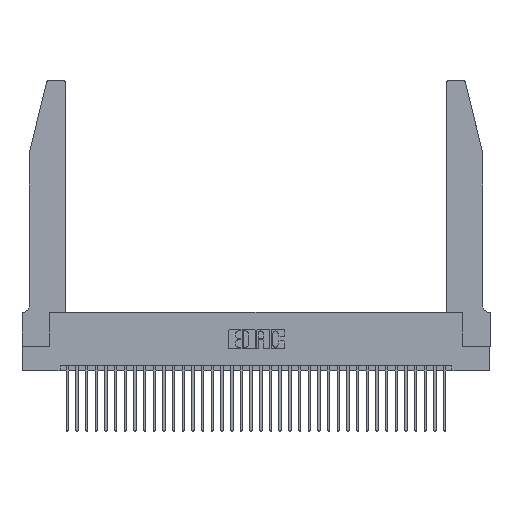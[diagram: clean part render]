
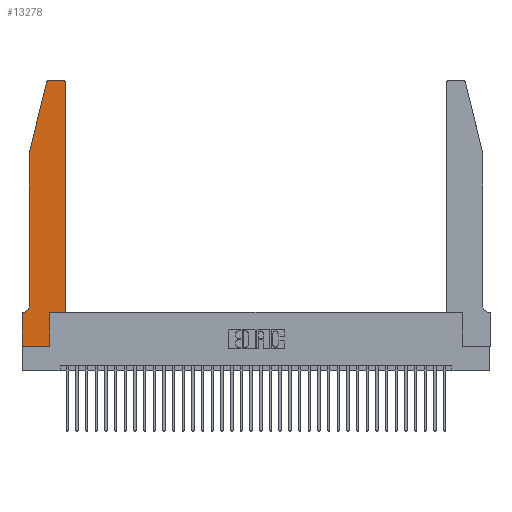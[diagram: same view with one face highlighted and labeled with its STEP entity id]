
A CAD part, top view. The second image highlights one B-rep face of the part: STEP entity #13278.
In plain terms, the highlighted planar face has unit normal (0, 0, 1).
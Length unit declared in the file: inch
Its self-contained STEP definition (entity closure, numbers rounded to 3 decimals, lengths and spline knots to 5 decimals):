
#211 = VERTEX_POINT ( 'NONE', #30569 ) ;
#705 = CARTESIAN_POINT ( 'NONE',  ( 0., 0.35, 0.37 ) ) ;
#905 = CIRCLE ( 'NONE', #9524, 0.03 ) ;
#2396 = VERTEX_POINT ( 'NONE', #23464 ) ;
#2611 = LINE ( 'NONE', #6939, #23363 ) ;
#3574 = DIRECTION ( 'NONE',  ( 1., 0., 0. ) ) ;
#3720 = CARTESIAN_POINT ( 'NONE',  ( 0.4505, 0.35, 0.37 ) ) ;
#4572 = CARTESIAN_POINT ( 'NONE',  ( 0.25487, 2.72718, 0.37 ) ) ;
#5302 = VECTOR ( 'NONE', #16396, 39.37008 ) ;
#5858 = ORIENTED_EDGE ( 'NONE', *, *, #14183, .T. ) ;
#5920 = DIRECTION ( 'NONE',  ( 0., -1., 0. ) ) ;
#6139 = VERTEX_POINT ( 'NONE', #10000 ) ;
#6207 = VERTEX_POINT ( 'NONE', #4572 ) ;
#6269 = ORIENTED_EDGE ( 'NONE', *, *, #28513, .T. ) ;
#6939 = CARTESIAN_POINT ( 'NONE',  ( 0.4505, 0.35, 0.37 ) ) ;
#7108 = CARTESIAN_POINT ( 'NONE',  ( 0.4505, 0.35, 0.37 ) ) ;
#8705 = CARTESIAN_POINT ( 'NONE',  ( 0.4205, 2.72, 0.37 ) ) ;
#8706 = ORIENTED_EDGE ( 'NONE', *, *, #33231, .T. ) ;
#9193 = CARTESIAN_POINT ( 'NONE',  ( 0., 0., 0.37 ) ) ;
#9355 = CARTESIAN_POINT ( 'NONE',  ( 0.0055, 0.42, 0.37 ) ) ;
#9356 = CARTESIAN_POINT ( 'NONE',  ( 0.0755, 0.35, 0.37 ) ) ;
#9372 = ORIENTED_EDGE ( 'NONE', *, *, #35057, .T. ) ;
#9524 = AXIS2_PLACEMENT_3D ( 'NONE', #8705, #28424, #11542 ) ;
#9559 = DIRECTION ( 'NONE',  ( 0., -1., 0. ) ) ;
#9807 = VECTOR ( 'NONE', #5920, 39.37008 ) ;
#9997 = ORIENTED_EDGE ( 'NONE', *, *, #34305, .T. ) ;
#10000 = CARTESIAN_POINT ( 'NONE',  ( 0.4205, 2.75, 0.37 ) ) ;
#10575 = AXIS2_PLACEMENT_3D ( 'NONE', #705, #20532, #3574 ) ;
#10617 = CARTESIAN_POINT ( 'NONE',  ( 0.0055, 0.35, 0.37 ) ) ;
#10676 = VECTOR ( 'NONE', #29882, 39.37008 ) ;
#10998 = VECTOR ( 'NONE', #12276, 39.37008 ) ;
#11542 = DIRECTION ( 'NONE',  ( 1., 0., 0. ) ) ;
#11963 = LINE ( 'NONE', #33065, #26085 ) ;
#12200 = DIRECTION ( 'NONE',  ( -1., 0., 0. ) ) ;
#12276 = DIRECTION ( 'NONE',  ( 0., 1., 0. ) ) ;
#12331 = ORIENTED_EDGE ( 'NONE', *, *, #19275, .T. ) ;
#12383 = LINE ( 'NONE', #9356, #27407 ) ;
#12511 = ORIENTED_EDGE ( 'NONE', *, *, #20801, .T. ) ;
#13278 = ADVANCED_FACE ( 'NONE', ( #25764 ), #31632, .T. ) ;
#13714 = ORIENTED_EDGE ( 'NONE', *, *, #14880, .T. ) ;
#13717 = CARTESIAN_POINT ( 'NONE',  ( 0.284, 2.72, 0.37 ) ) ;
#14183 = EDGE_CURVE ( 'NONE', #6139, #31947, #18225, .T. ) ;
#14285 = EDGE_LOOP ( 'NONE', ( #5858, #9997, #12511, #12331, #28300, #33440, #23217, #13714, #6269, #9372, #17600, #8706 ) ) ;
#14880 = EDGE_CURVE ( 'NONE', #26046, #22885, #11963, .T. ) ;
#15462 = VECTOR ( 'NONE', #23461, 39.37008 ) ;
#15793 = CARTESIAN_POINT ( 'NONE',  ( 0.284, 2.75, 0.37 ) ) ;
#15962 = EDGE_CURVE ( 'NONE', #35844, #27757, #2611, .T. ) ;
#16319 = VERTEX_POINT ( 'NONE', #28370 ) ;
#16396 = DIRECTION ( 'NONE',  ( -0.239, -0.971, 0. ) ) ;
#16585 = DIRECTION ( 'NONE',  ( 1., 0., 0. ) ) ;
#17018 = LINE ( 'NONE', #23648, #31023 ) ;
#17600 = ORIENTED_EDGE ( 'NONE', *, *, #15962, .T. ) ;
#18073 = EDGE_CURVE ( 'NONE', #2396, #26046, #17018, .T. ) ;
#18225 = LINE ( 'NONE', #27101, #10676 ) ;
#19275 = EDGE_CURVE ( 'NONE', #16319, #27508, #32242, .T. ) ;
#19389 = EDGE_CURVE ( 'NONE', #27508, #34283, #19570, .T. ) ;
#19570 = CIRCLE ( 'NONE', #25615, 0.07 ) ;
#20532 = DIRECTION ( 'NONE',  ( 0., 0., 1. ) ) ;
#20801 = EDGE_CURVE ( 'NONE', #6207, #16319, #35178, .T. ) ;
#21952 = CARTESIAN_POINT ( 'NONE',  ( 0.0755, 2., 0.37 ) ) ;
#22581 = AXIS2_PLACEMENT_3D ( 'NONE', #13717, #33326, #16585 ) ;
#22885 = VERTEX_POINT ( 'NONE', #31319 ) ;
#23217 = ORIENTED_EDGE ( 'NONE', *, *, #18073, .T. ) ;
#23363 = VECTOR ( 'NONE', #32264, 39.37008 ) ;
#23461 = DIRECTION ( 'NONE',  ( 1., 0., 0. ) ) ;
#23464 = CARTESIAN_POINT ( 'NONE',  ( 0., 0.35, 0.37 ) ) ;
#23648 = CARTESIAN_POINT ( 'NONE',  ( 0., 0., 0.37 ) ) ;
#25582 = CIRCLE ( 'NONE', #22581, 0.03 ) ;
#25615 = AXIS2_PLACEMENT_3D ( 'NONE', #9355, #29084, #12200 ) ;
#25658 = CARTESIAN_POINT ( 'NONE',  ( 0.0755, 2., 0.37 ) ) ;
#25764 = FACE_OUTER_BOUND ( 'NONE', #14285, .T. ) ;
#26024 = LINE ( 'NONE', #31929, #10998 ) ;
#26046 = VERTEX_POINT ( 'NONE', #9193 ) ;
#26085 = VECTOR ( 'NONE', #35870, 39.37008 ) ;
#26280 = DIRECTION ( 'NONE',  ( -1., 0., 0. ) ) ;
#27101 = CARTESIAN_POINT ( 'NONE',  ( 0.2605, 2.75, 0.37 ) ) ;
#27407 = VECTOR ( 'NONE', #26280, 39.37008 ) ;
#27508 = VERTEX_POINT ( 'NONE', #35775 ) ;
#27757 = VERTEX_POINT ( 'NONE', #31624 ) ;
#27794 = EDGE_CURVE ( 'NONE', #34283, #2396, #12383, .T. ) ;
#28300 = ORIENTED_EDGE ( 'NONE', *, *, #19389, .T. ) ;
#28370 = CARTESIAN_POINT ( 'NONE',  ( 0.0755, 2., 0.37 ) ) ;
#28424 = DIRECTION ( 'NONE',  ( 0., 0., 1. ) ) ;
#28513 = EDGE_CURVE ( 'NONE', #22885, #211, #26024, .T. ) ;
#29084 = DIRECTION ( 'NONE',  ( 0., 0., -1. ) ) ;
#29882 = DIRECTION ( 'NONE',  ( -1., 0., 0. ) ) ;
#30402 = LINE ( 'NONE', #3720, #15462 ) ;
#30569 = CARTESIAN_POINT ( 'NONE',  ( 0.2865, 0.35, 0.37 ) ) ;
#31023 = VECTOR ( 'NONE', #9559, 39.37008 ) ;
#31319 = CARTESIAN_POINT ( 'NONE',  ( 0.2865, 0., 0.37 ) ) ;
#31624 = CARTESIAN_POINT ( 'NONE',  ( 0.4505, 2.72, 0.37 ) ) ;
#31632 = PLANE ( 'NONE',  #10575 ) ;
#31929 = CARTESIAN_POINT ( 'NONE',  ( 0.2865, 0.35, 0.37 ) ) ;
#31947 = VERTEX_POINT ( 'NONE', #15793 ) ;
#32242 = LINE ( 'NONE', #25658, #9807 ) ;
#32264 = DIRECTION ( 'NONE',  ( 0., 1., 0. ) ) ;
#33065 = CARTESIAN_POINT ( 'NONE',  ( 0., 0., 0.37 ) ) ;
#33231 = EDGE_CURVE ( 'NONE', #27757, #6139, #905, .T. ) ;
#33326 = DIRECTION ( 'NONE',  ( 0., 0., 1. ) ) ;
#33440 = ORIENTED_EDGE ( 'NONE', *, *, #27794, .T. ) ;
#34283 = VERTEX_POINT ( 'NONE', #10617 ) ;
#34305 = EDGE_CURVE ( 'NONE', #31947, #6207, #25582, .T. ) ;
#35057 = EDGE_CURVE ( 'NONE', #211, #35844, #30402, .T. ) ;
#35178 = LINE ( 'NONE', #21952, #5302 ) ;
#35775 = CARTESIAN_POINT ( 'NONE',  ( 0.0755, 0.42, 0.37 ) ) ;
#35844 = VERTEX_POINT ( 'NONE', #7108 ) ;
#35870 = DIRECTION ( 'NONE',  ( 1., 0., 0. ) ) ;
